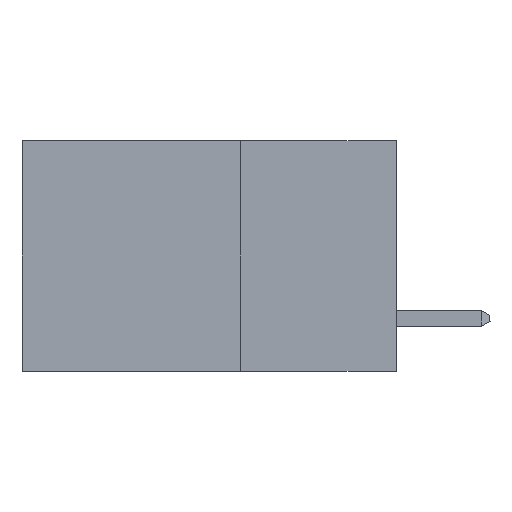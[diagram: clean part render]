
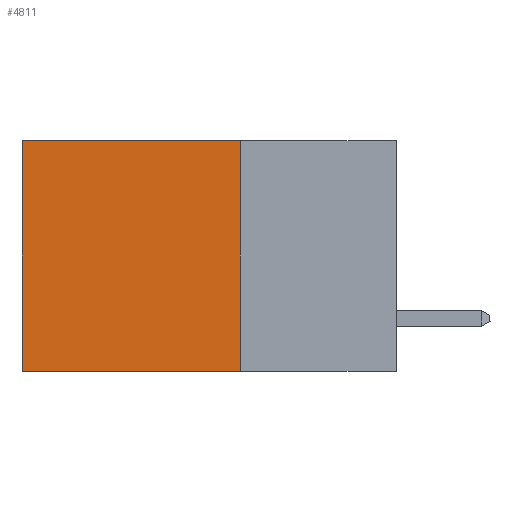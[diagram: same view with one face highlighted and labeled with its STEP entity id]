
A CAD part, left-side view. The second image highlights one B-rep face of the part: STEP entity #4811.
In plain terms, the highlighted planar face has unit normal (-1, 0, 0).
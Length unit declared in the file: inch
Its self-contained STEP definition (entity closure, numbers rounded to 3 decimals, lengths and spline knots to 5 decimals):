
#164 = AXIS2_PLACEMENT_3D ( 'NONE', #6479, #2399, #7910 ) ;
#197 = VECTOR ( 'NONE', #15736, 39.37008 ) ;
#216 = LINE ( 'NONE', #10326, #11139 ) ;
#485 = ORIENTED_EDGE ( 'NONE', *, *, #11110, .T. ) ;
#2399 = DIRECTION ( 'NONE',  ( 1., 0., 0. ) ) ;
#3002 = VERTEX_POINT ( 'NONE', #3961 ) ;
#3301 = VERTEX_POINT ( 'NONE', #13436 ) ;
#3576 = EDGE_CURVE ( 'NONE', #13874, #3002, #8207, .T. ) ;
#3961 = CARTESIAN_POINT ( 'NONE',  ( 0.298, 0.25, -0.37 ) ) ;
#4054 = VECTOR ( 'NONE', #15143, 39.37008 ) ;
#4387 = CARTESIAN_POINT ( 'NONE',  ( 0.298, 0.6, -0.37 ) ) ;
#4621 = EDGE_LOOP ( 'NONE', ( #485, #10476, #10928, #7431 ) ) ;
#4811 = ADVANCED_FACE ( 'NONE', ( #6145 ), #18250, .F. ) ;
#6145 = FACE_OUTER_BOUND ( 'NONE', #4621, .T. ) ;
#6456 = CARTESIAN_POINT ( 'NONE',  ( 0.298, 0.25, 0. ) ) ;
#6479 = CARTESIAN_POINT ( 'NONE',  ( 0.298, 0.25, 0. ) ) ;
#6982 = CARTESIAN_POINT ( 'NONE',  ( 0.298, 0.25, 0. ) ) ;
#7431 = ORIENTED_EDGE ( 'NONE', *, *, #13475, .T. ) ;
#7910 = DIRECTION ( 'NONE',  ( 0., 0., -1. ) ) ;
#8207 = LINE ( 'NONE', #6456, #197 ) ;
#8808 = VERTEX_POINT ( 'NONE', #4387 ) ;
#9387 = VECTOR ( 'NONE', #18030, 39.37008 ) ;
#9568 = CARTESIAN_POINT ( 'NONE',  ( 0.298, 0.6, 0. ) ) ;
#10326 = CARTESIAN_POINT ( 'NONE',  ( 0.298, 0.25, 0. ) ) ;
#10476 = ORIENTED_EDGE ( 'NONE', *, *, #17376, .F. ) ;
#10928 = ORIENTED_EDGE ( 'NONE', *, *, #3576, .F. ) ;
#11110 = EDGE_CURVE ( 'NONE', #3301, #8808, #13220, .T. ) ;
#11139 = VECTOR ( 'NONE', #11808, 39.37008 ) ;
#11765 = LINE ( 'NONE', #12419, #4054 ) ;
#11808 = DIRECTION ( 'NONE',  ( 0., 1., 0. ) ) ;
#12419 = CARTESIAN_POINT ( 'NONE',  ( 0.298, 0.25, -0.37 ) ) ;
#13220 = LINE ( 'NONE', #9568, #9387 ) ;
#13436 = CARTESIAN_POINT ( 'NONE',  ( 0.298, 0.6, 0. ) ) ;
#13475 = EDGE_CURVE ( 'NONE', #13874, #3301, #216, .T. ) ;
#13874 = VERTEX_POINT ( 'NONE', #6982 ) ;
#15143 = DIRECTION ( 'NONE',  ( 0., 1., 0. ) ) ;
#15736 = DIRECTION ( 'NONE',  ( 0., 0., -1. ) ) ;
#17376 = EDGE_CURVE ( 'NONE', #3002, #8808, #11765, .T. ) ;
#18030 = DIRECTION ( 'NONE',  ( 0., 0., -1. ) ) ;
#18250 = PLANE ( 'NONE',  #164 ) ;
